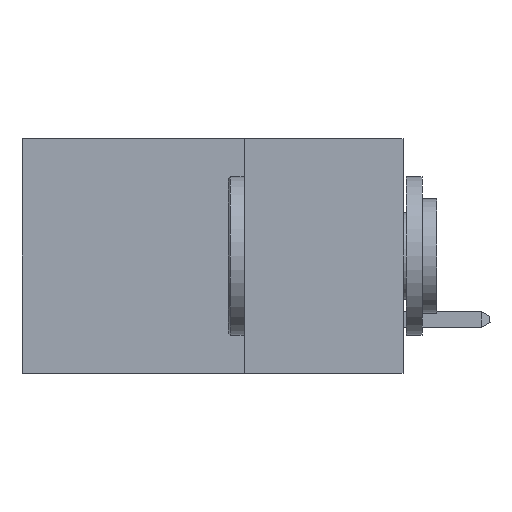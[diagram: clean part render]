
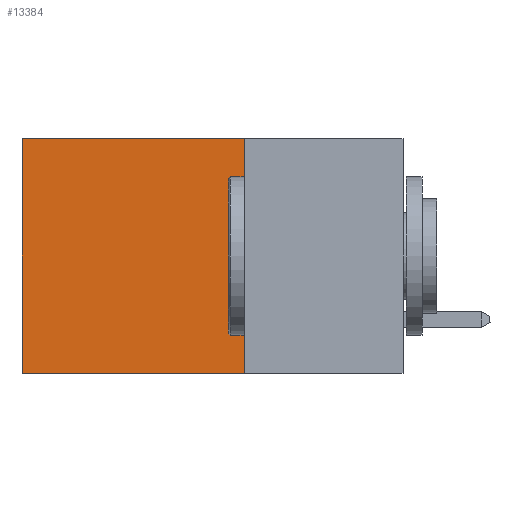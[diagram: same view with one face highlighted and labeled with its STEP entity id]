
A CAD part, left-side view. The second image highlights one B-rep face of the part: STEP entity #13384.
In plain terms, the highlighted planar face has unit normal (-1, 0, 0).
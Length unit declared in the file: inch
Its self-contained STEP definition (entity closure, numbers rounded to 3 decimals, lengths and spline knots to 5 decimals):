
#2782 = VERTEX_POINT ( 'NONE', #11260 ) ;
#3197 = DIRECTION ( 'NONE',  ( 0., 0., -1. ) ) ;
#3748 = DIRECTION ( 'NONE',  ( 0., 1., 0. ) ) ;
#4639 = AXIS2_PLACEMENT_3D ( 'NONE', #35733, #15315, #18750 ) ;
#5377 = EDGE_LOOP ( 'NONE', ( #30061, #10076, #5956, #35590 ) ) ;
#5518 = CARTESIAN_POINT ( 'NONE',  ( 0.2875, 0.6, -0.37 ) ) ;
#5956 = ORIENTED_EDGE ( 'NONE', *, *, #12720, .F. ) ;
#6030 = VECTOR ( 'NONE', #32626, 39.37008 ) ;
#8868 = LINE ( 'NONE', #33661, #43980 ) ;
#9832 = EDGE_CURVE ( 'NONE', #2782, #34540, #30976, .T. ) ;
#10076 = ORIENTED_EDGE ( 'NONE', *, *, #14157, .F. ) ;
#11260 = CARTESIAN_POINT ( 'NONE',  ( 0.2875, 0.6, 0. ) ) ;
#12720 = EDGE_CURVE ( 'NONE', #36872, #42457, #8868, .T. ) ;
#13384 = ADVANCED_FACE ( 'NONE', ( #16757 ), #22012, .F. ) ;
#14157 = EDGE_CURVE ( 'NONE', #42457, #34540, #34192, .T. ) ;
#14572 = DIRECTION ( 'NONE',  ( 0., 1., 0. ) ) ;
#15315 = DIRECTION ( 'NONE',  ( 1., 0., 0. ) ) ;
#16757 = FACE_OUTER_BOUND ( 'NONE', #5377, .T. ) ;
#18750 = DIRECTION ( 'NONE',  ( 0., 0., -1. ) ) ;
#22012 = PLANE ( 'NONE',  #4639 ) ;
#22580 = EDGE_CURVE ( 'NONE', #36872, #2782, #34648, .T. ) ;
#23438 = VECTOR ( 'NONE', #14572, 39.37008 ) ;
#24062 = CARTESIAN_POINT ( 'NONE',  ( 0.2875, 0.25, -0.37 ) ) ;
#30061 = ORIENTED_EDGE ( 'NONE', *, *, #9832, .T. ) ;
#30976 = LINE ( 'NONE', #32005, #6030 ) ;
#32005 = CARTESIAN_POINT ( 'NONE',  ( 0.2875, 0.6, 0. ) ) ;
#32626 = DIRECTION ( 'NONE',  ( 0., 0., -1. ) ) ;
#33661 = CARTESIAN_POINT ( 'NONE',  ( 0.2875, 0.25, 0. ) ) ;
#34192 = LINE ( 'NONE', #24062, #42782 ) ;
#34540 = VERTEX_POINT ( 'NONE', #5518 ) ;
#34648 = LINE ( 'NONE', #34967, #23438 ) ;
#34967 = CARTESIAN_POINT ( 'NONE',  ( 0.2875, 0.25, 0. ) ) ;
#35590 = ORIENTED_EDGE ( 'NONE', *, *, #22580, .T. ) ;
#35733 = CARTESIAN_POINT ( 'NONE',  ( 0.2875, 0.25, 0. ) ) ;
#36872 = VERTEX_POINT ( 'NONE', #39493 ) ;
#39493 = CARTESIAN_POINT ( 'NONE',  ( 0.2875, 0.25, 0. ) ) ;
#42457 = VERTEX_POINT ( 'NONE', #43937 ) ;
#42782 = VECTOR ( 'NONE', #3748, 39.37008 ) ;
#43937 = CARTESIAN_POINT ( 'NONE',  ( 0.2875, 0.25, -0.37 ) ) ;
#43980 = VECTOR ( 'NONE', #3197, 39.37008 ) ;
